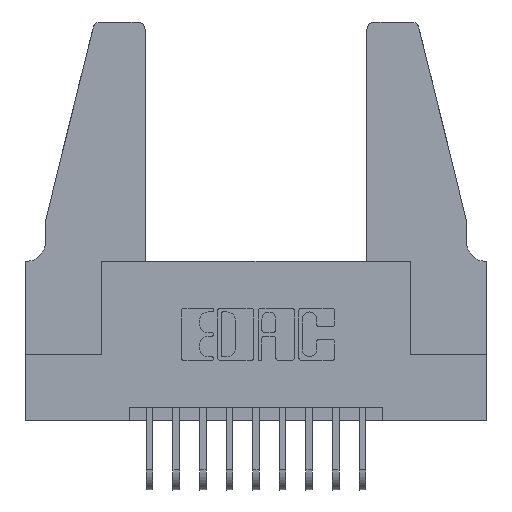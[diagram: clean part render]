
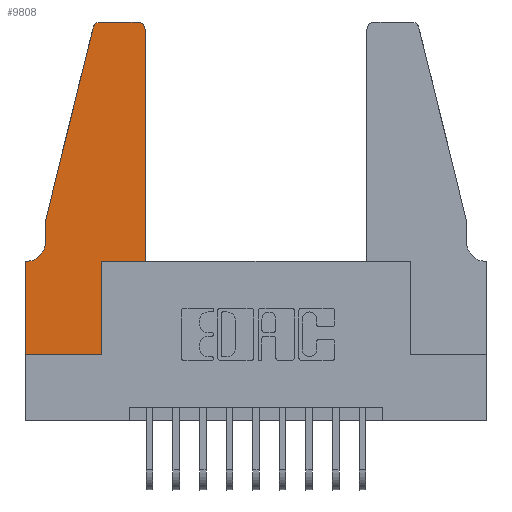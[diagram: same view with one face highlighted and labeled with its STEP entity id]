
A CAD part, top view. The second image highlights one B-rep face of the part: STEP entity #9808.
In plain terms, the highlighted planar face has unit normal (0, 0, 1).
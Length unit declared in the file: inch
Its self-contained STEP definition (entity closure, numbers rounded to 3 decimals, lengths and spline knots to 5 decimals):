
#34 = ORIENTED_EDGE ( 'NONE', *, *, #13823, .T. ) ;
#63 = CARTESIAN_POINT ( 'NONE',  ( 0., 0., 0.37 ) ) ;
#204 = LINE ( 'NONE', #1281, #5022 ) ;
#684 = CIRCLE ( 'NONE', #11931, 0.03 ) ;
#824 = DIRECTION ( 'NONE',  ( 0., 0., 1. ) ) ;
#872 = DIRECTION ( 'NONE',  ( 0., -1., 0. ) ) ;
#1281 = CARTESIAN_POINT ( 'NONE',  ( 0., 0., 0.37 ) ) ;
#1665 = ORIENTED_EDGE ( 'NONE', *, *, #8109, .T. ) ;
#1760 = EDGE_CURVE ( 'NONE', #4608, #13707, #5261, .T. ) ;
#1762 = LINE ( 'NONE', #63, #4174 ) ;
#2050 = AXIS2_PLACEMENT_3D ( 'NONE', #11316, #14946, #12544 ) ;
#2051 = VERTEX_POINT ( 'NONE', #2198 ) ;
#2059 = CARTESIAN_POINT ( 'NONE',  ( 0.0755, 0.35, 0.37 ) ) ;
#2118 = CARTESIAN_POINT ( 'NONE',  ( 0.284, 1.22, 0.37 ) ) ;
#2129 = DIRECTION ( 'NONE',  ( -1., 0., 0. ) ) ;
#2198 = CARTESIAN_POINT ( 'NONE',  ( 0.0055, 0.35, 0.37 ) ) ;
#2251 = ORIENTED_EDGE ( 'NONE', *, *, #3452, .T. ) ;
#2394 = CARTESIAN_POINT ( 'NONE',  ( 0.4505, 0.35, 0.37 ) ) ;
#2519 = CARTESIAN_POINT ( 'NONE',  ( 0.2865, 0.35, 0.37 ) ) ;
#2546 = AXIS2_PLACEMENT_3D ( 'NONE', #7488, #5230, #11052 ) ;
#2962 = CARTESIAN_POINT ( 'NONE',  ( 0.2865, 0.35, 0.37 ) ) ;
#3070 = EDGE_CURVE ( 'NONE', #4388, #8108, #6698, .T. ) ;
#3173 = CARTESIAN_POINT ( 'NONE',  ( 0.0755, 0.5, 0.37 ) ) ;
#3233 = LINE ( 'NONE', #13560, #3979 ) ;
#3252 = EDGE_LOOP ( 'NONE', ( #14988, #34, #13096, #15296, #3566, #9627, #14367, #2251, #4465, #1665, #6353, #4695 ) ) ;
#3370 = FACE_OUTER_BOUND ( 'NONE', #3252, .T. ) ;
#3396 = DIRECTION ( 'NONE',  ( 1., 0., 0. ) ) ;
#3433 = CARTESIAN_POINT ( 'NONE',  ( 0.4205, 1.25, 0.37 ) ) ;
#3452 = EDGE_CURVE ( 'NONE', #15295, #4388, #204, .T. ) ;
#3456 = CARTESIAN_POINT ( 'NONE',  ( 0.0755, 0.5, 0.37 ) ) ;
#3465 = LINE ( 'NONE', #3173, #8265 ) ;
#3480 = CARTESIAN_POINT ( 'NONE',  ( 0.2865, 0., 0.37 ) ) ;
#3566 = ORIENTED_EDGE ( 'NONE', *, *, #10963, .T. ) ;
#3979 = VECTOR ( 'NONE', #5086, 39.37008 ) ;
#4174 = VECTOR ( 'NONE', #872, 39.37008 ) ;
#4180 = VERTEX_POINT ( 'NONE', #6587 ) ;
#4341 = VECTOR ( 'NONE', #8552, 39.37008 ) ;
#4365 = CARTESIAN_POINT ( 'NONE',  ( 0.284, 1.25, 0.37 ) ) ;
#4388 = VERTEX_POINT ( 'NONE', #3480 ) ;
#4465 = ORIENTED_EDGE ( 'NONE', *, *, #3070, .T. ) ;
#4608 = VERTEX_POINT ( 'NONE', #14507 ) ;
#4658 = CARTESIAN_POINT ( 'NONE',  ( 0., 0.35, 0.37 ) ) ;
#4695 = ORIENTED_EDGE ( 'NONE', *, *, #6880, .T. ) ;
#4718 = AXIS2_PLACEMENT_3D ( 'NONE', #11505, #824, #10273 ) ;
#4725 = CARTESIAN_POINT ( 'NONE',  ( 0.4505, 1.22, 0.37 ) ) ;
#4759 = VECTOR ( 'NONE', #10434, 39.37008 ) ;
#5022 = VECTOR ( 'NONE', #10727, 39.37008 ) ;
#5040 = VECTOR ( 'NONE', #14878, 39.37008 ) ;
#5086 = DIRECTION ( 'NONE',  ( 1., 0., 0. ) ) ;
#5230 = DIRECTION ( 'NONE',  ( 0., 0., -1. ) ) ;
#5261 = LINE ( 'NONE', #3456, #4341 ) ;
#5382 = VERTEX_POINT ( 'NONE', #6287 ) ;
#5710 = CARTESIAN_POINT ( 'NONE',  ( 0.2605, 1.25, 0.37 ) ) ;
#5746 = DIRECTION ( 'NONE',  ( 0., 0., 1. ) ) ;
#6287 = CARTESIAN_POINT ( 'NONE',  ( 0.25487, 1.22718, 0.37 ) ) ;
#6353 = ORIENTED_EDGE ( 'NONE', *, *, #7263, .T. ) ;
#6587 = CARTESIAN_POINT ( 'NONE',  ( 0.4505, 0.35, 0.37 ) ) ;
#6610 = CIRCLE ( 'NONE', #2050, 0.03 ) ;
#6698 = LINE ( 'NONE', #2962, #5040 ) ;
#6744 = DIRECTION ( 'NONE',  ( -0.239, -0.971, 0. ) ) ;
#6880 = EDGE_CURVE ( 'NONE', #14286, #12833, #6610, .T. ) ;
#6905 = VERTEX_POINT ( 'NONE', #4365 ) ;
#6913 = EDGE_CURVE ( 'NONE', #5382, #4608, #3465, .T. ) ;
#7220 = EDGE_CURVE ( 'NONE', #12833, #6905, #7702, .T. ) ;
#7263 = EDGE_CURVE ( 'NONE', #4180, #14286, #13631, .T. ) ;
#7488 = CARTESIAN_POINT ( 'NONE',  ( 0.0055, 0.42, 0.37 ) ) ;
#7702 = LINE ( 'NONE', #5710, #8614 ) ;
#7799 = EDGE_CURVE ( 'NONE', #14854, #15295, #1762, .T. ) ;
#7844 = EDGE_CURVE ( 'NONE', #2051, #14854, #7864, .T. ) ;
#7864 = LINE ( 'NONE', #2059, #13595 ) ;
#8108 = VERTEX_POINT ( 'NONE', #2519 ) ;
#8109 = EDGE_CURVE ( 'NONE', #8108, #4180, #3233, .T. ) ;
#8265 = VECTOR ( 'NONE', #6744, 39.37008 ) ;
#8552 = DIRECTION ( 'NONE',  ( 0., -1., 0. ) ) ;
#8614 = VECTOR ( 'NONE', #2129, 39.37008 ) ;
#9231 = PLANE ( 'NONE',  #4718 ) ;
#9533 = DIRECTION ( 'NONE',  ( -1., 0., 0. ) ) ;
#9627 = ORIENTED_EDGE ( 'NONE', *, *, #7844, .T. ) ;
#9808 = ADVANCED_FACE ( 'NONE', ( #3370 ), #9231, .T. ) ;
#10273 = DIRECTION ( 'NONE',  ( 1., 0., 0. ) ) ;
#10434 = DIRECTION ( 'NONE',  ( 0., 1., 0. ) ) ;
#10727 = DIRECTION ( 'NONE',  ( 1., 0., 0. ) ) ;
#10963 = EDGE_CURVE ( 'NONE', #13707, #2051, #13149, .T. ) ;
#11052 = DIRECTION ( 'NONE',  ( -1., 0., 0. ) ) ;
#11316 = CARTESIAN_POINT ( 'NONE',  ( 0.4205, 1.22, 0.37 ) ) ;
#11505 = CARTESIAN_POINT ( 'NONE',  ( 0., 0.35, 0.37 ) ) ;
#11570 = CARTESIAN_POINT ( 'NONE',  ( 0., 0., 0.37 ) ) ;
#11931 = AXIS2_PLACEMENT_3D ( 'NONE', #2118, #5746, #3396 ) ;
#12544 = DIRECTION ( 'NONE',  ( 1., 0., 0. ) ) ;
#12833 = VERTEX_POINT ( 'NONE', #3433 ) ;
#13096 = ORIENTED_EDGE ( 'NONE', *, *, #6913, .T. ) ;
#13149 = CIRCLE ( 'NONE', #2546, 0.07 ) ;
#13260 = CARTESIAN_POINT ( 'NONE',  ( 0.0755, 0.42, 0.37 ) ) ;
#13560 = CARTESIAN_POINT ( 'NONE',  ( 0.4505, 0.35, 0.37 ) ) ;
#13595 = VECTOR ( 'NONE', #9533, 39.37008 ) ;
#13631 = LINE ( 'NONE', #2394, #4759 ) ;
#13707 = VERTEX_POINT ( 'NONE', #13260 ) ;
#13823 = EDGE_CURVE ( 'NONE', #6905, #5382, #684, .T. ) ;
#14286 = VERTEX_POINT ( 'NONE', #4725 ) ;
#14367 = ORIENTED_EDGE ( 'NONE', *, *, #7799, .T. ) ;
#14507 = CARTESIAN_POINT ( 'NONE',  ( 0.0755, 0.5, 0.37 ) ) ;
#14854 = VERTEX_POINT ( 'NONE', #4658 ) ;
#14878 = DIRECTION ( 'NONE',  ( 0., 1., 0. ) ) ;
#14946 = DIRECTION ( 'NONE',  ( 0., 0., 1. ) ) ;
#14988 = ORIENTED_EDGE ( 'NONE', *, *, #7220, .T. ) ;
#15295 = VERTEX_POINT ( 'NONE', #11570 ) ;
#15296 = ORIENTED_EDGE ( 'NONE', *, *, #1760, .T. ) ;
